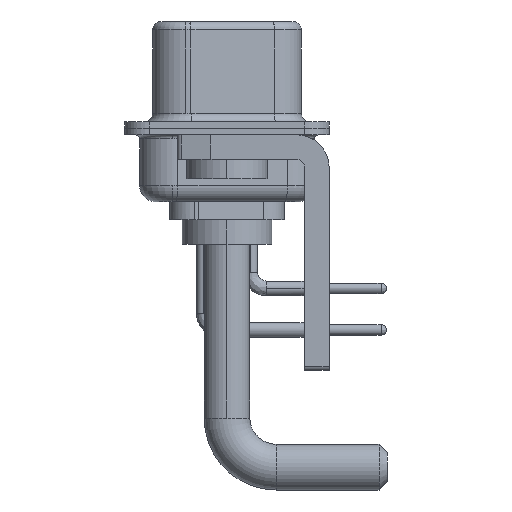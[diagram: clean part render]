
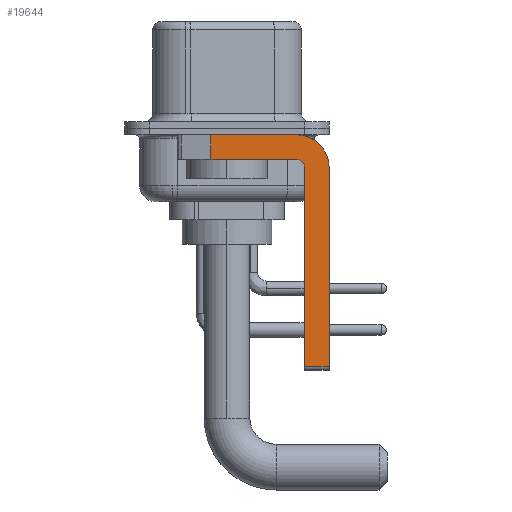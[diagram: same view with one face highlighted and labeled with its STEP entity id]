
A CAD part, left-side view. The second image highlights one B-rep face of the part: STEP entity #19644.
In plain terms, the highlighted planar face has unit normal (-1, 0, 0).
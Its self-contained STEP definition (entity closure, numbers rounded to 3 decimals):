
#435 = EDGE_CURVE ( 'NONE', #19456, #8116, #25133, .T. ) ;
#2559 = VECTOR ( 'NONE', #19990, 1000. ) ;
#3927 = VECTOR ( 'NONE', #10983, 1000. ) ;
#4371 = ORIENTED_EDGE ( 'NONE', *, *, #7470, .F. ) ;
#4848 = CARTESIAN_POINT ( 'NONE',  ( -2.9, 0.978, -1.9 ) ) ;
#5889 = ORIENTED_EDGE ( 'NONE', *, *, #10657, .F. ) ;
#6012 = VERTEX_POINT ( 'NONE', #29115 ) ;
#6189 = ORIENTED_EDGE ( 'NONE', *, *, #15698, .T. ) ;
#6283 = CARTESIAN_POINT ( 'NONE',  ( -2.9, -4.25, -2.4 ) ) ;
#6360 = CARTESIAN_POINT ( 'NONE',  ( -2.9, -4.25, -1.9 ) ) ;
#6817 = CARTESIAN_POINT ( 'NONE',  ( -2.9, 3., -0.4 ) ) ;
#7470 = EDGE_CURVE ( 'NONE', #16009, #6012, #26319, .T. ) ;
#7789 = CARTESIAN_POINT ( 'NONE',  ( -2.9, 0.978, -0.4 ) ) ;
#7840 = DIRECTION ( 'NONE',  ( 0., 0., -1. ) ) ;
#8116 = VERTEX_POINT ( 'NONE', #4848 ) ;
#10076 = CARTESIAN_POINT ( 'NONE',  ( -2.9, -6.25, -2.4 ) ) ;
#10466 = DIRECTION ( 'NONE',  ( 1., 0., 0. ) ) ;
#10657 = EDGE_CURVE ( 'NONE', #26002, #23717, #16433, .T. ) ;
#10983 = DIRECTION ( 'NONE',  ( 0., -1., 0. ) ) ;
#11488 = VERTEX_POINT ( 'NONE', #29177 ) ;
#11532 = EDGE_CURVE ( 'NONE', #23717, #8116, #26653, .T. ) ;
#11930 = VECTOR ( 'NONE', #15772, 1000. ) ;
#12250 = CIRCLE ( 'NONE', #28895, 2. ) ;
#13833 = DIRECTION ( 'NONE',  ( 0., 0., -1. ) ) ;
#13834 = CARTESIAN_POINT ( 'NONE',  ( -2.9, -4.25, -1.9 ) ) ;
#14241 = ORIENTED_EDGE ( 'NONE', *, *, #27451, .F. ) ;
#14775 = ORIENTED_EDGE ( 'NONE', *, *, #435, .T. ) ;
#15392 = LINE ( 'NONE', #6817, #2559 ) ;
#15698 = EDGE_CURVE ( 'NONE', #11488, #6012, #17546, .T. ) ;
#15759 = EDGE_LOOP ( 'NONE', ( #19778, #14775, #26645, #5889, #14241, #6189, #4371, #21553 ) ) ;
#15764 = CARTESIAN_POINT ( 'NONE',  ( -2.9, -4.25, -0.4 ) ) ;
#15772 = DIRECTION ( 'NONE',  ( 0., 1., 0. ) ) ;
#16009 = VERTEX_POINT ( 'NONE', #19984 ) ;
#16433 = CIRCLE ( 'NONE', #23567, 0.5 ) ;
#17245 = CARTESIAN_POINT ( 'NONE',  ( -2.9, -4.25, -14.55 ) ) ;
#17253 = CARTESIAN_POINT ( 'NONE',  ( -2.9, -4.75, -14.8 ) ) ;
#17546 = LINE ( 'NONE', #17245, #3927 ) ;
#17779 = PLANE ( 'NONE',  #27874 ) ;
#18245 = EDGE_CURVE ( 'NONE', #19456, #20674, #15392, .T. ) ;
#19456 = VERTEX_POINT ( 'NONE', #7789 ) ;
#19644 = ADVANCED_FACE ( 'NONE', ( #20297 ), #17779, .F. ) ;
#19778 = ORIENTED_EDGE ( 'NONE', *, *, #18245, .F. ) ;
#19984 = CARTESIAN_POINT ( 'NONE',  ( -2.9, -6.25, -2.4 ) ) ;
#19990 = DIRECTION ( 'NONE',  ( 0., -1., 0. ) ) ;
#20297 = FACE_OUTER_BOUND ( 'NONE', #15759, .T. ) ;
#20674 = VERTEX_POINT ( 'NONE', #15764 ) ;
#20863 = LINE ( 'NONE', #17253, #25535 ) ;
#21107 = EDGE_CURVE ( 'NONE', #20674, #16009, #12250, .T. ) ;
#21553 = ORIENTED_EDGE ( 'NONE', *, *, #21107, .F. ) ;
#22744 = CARTESIAN_POINT ( 'NONE',  ( -2.9, 0.978, -1.9 ) ) ;
#23567 = AXIS2_PLACEMENT_3D ( 'NONE', #6283, #29096, #24475 ) ;
#23604 = VECTOR ( 'NONE', #7840, 1000. ) ;
#23717 = VERTEX_POINT ( 'NONE', #13834 ) ;
#24475 = DIRECTION ( 'NONE',  ( 0., 0., 1. ) ) ;
#25133 = LINE ( 'NONE', #22744, #28511 ) ;
#25535 = VECTOR ( 'NONE', #27733, 1000. ) ;
#26002 = VERTEX_POINT ( 'NONE', #27394 ) ;
#26319 = LINE ( 'NONE', #10076, #23604 ) ;
#26422 = DIRECTION ( 'NONE',  ( 0., 0., -1. ) ) ;
#26645 = ORIENTED_EDGE ( 'NONE', *, *, #11532, .F. ) ;
#26653 = LINE ( 'NONE', #6360, #11930 ) ;
#26865 = CARTESIAN_POINT ( 'NONE',  ( -2.9, -4.25, -2.4 ) ) ;
#27394 = CARTESIAN_POINT ( 'NONE',  ( -2.9, -4.75, -2.4 ) ) ;
#27451 = EDGE_CURVE ( 'NONE', #11488, #26002, #20863, .T. ) ;
#27733 = DIRECTION ( 'NONE',  ( 0., 0., 1. ) ) ;
#27874 = AXIS2_PLACEMENT_3D ( 'NONE', #26865, #29386, #29240 ) ;
#28511 = VECTOR ( 'NONE', #13833, 1000. ) ;
#28797 = CARTESIAN_POINT ( 'NONE',  ( -2.9, -4.25, -2.4 ) ) ;
#28895 = AXIS2_PLACEMENT_3D ( 'NONE', #28797, #10466, #26422 ) ;
#29096 = DIRECTION ( 'NONE',  ( -1., 0., 0. ) ) ;
#29115 = CARTESIAN_POINT ( 'NONE',  ( -2.9, -6.25, -14.55 ) ) ;
#29177 = CARTESIAN_POINT ( 'NONE',  ( -2.9, -4.75, -14.55 ) ) ;
#29240 = DIRECTION ( 'NONE',  ( 0., 0., -1. ) ) ;
#29386 = DIRECTION ( 'NONE',  ( 1., 0., 0. ) ) ;
